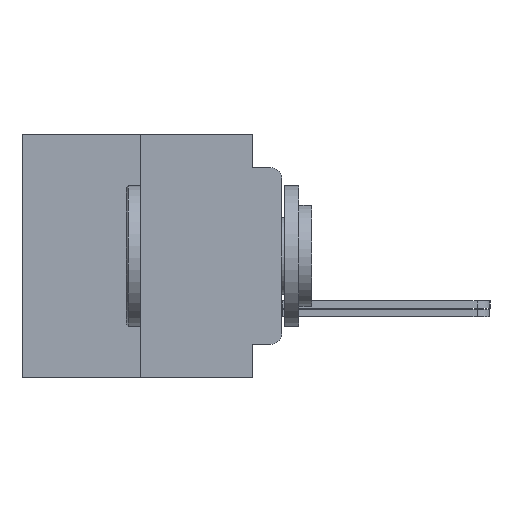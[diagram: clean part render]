
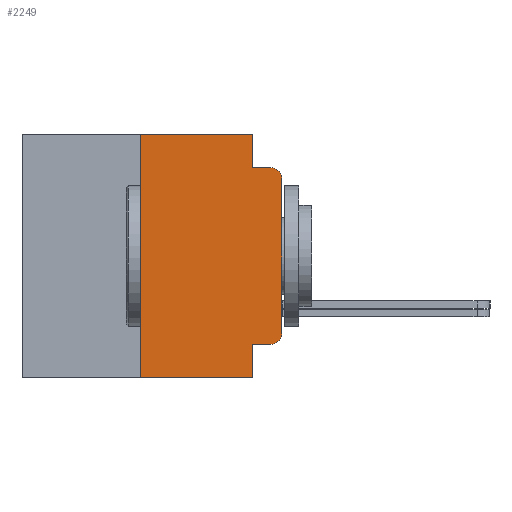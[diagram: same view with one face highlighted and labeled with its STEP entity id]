
A CAD part, left-side view. The second image highlights one B-rep face of the part: STEP entity #2249.
In plain terms, the highlighted planar face has unit normal (-1, 0, 0).
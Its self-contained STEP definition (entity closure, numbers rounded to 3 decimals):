
#635 = VECTOR ( 'NONE', #7273, 1000. ) ;
#1707 = CARTESIAN_POINT ( 'NONE',  ( -75.603, 0., -3.467 ) ) ;
#2099 = VERTEX_POINT ( 'NONE', #4735 ) ;
#2216 = VERTEX_POINT ( 'NONE', #3158 ) ;
#2249 = ADVANCED_FACE ( 'NONE', ( #16109 ), #23556, .F. ) ;
#3158 = CARTESIAN_POINT ( 'NONE',  ( -75.603, 0.508, 3.975 ) ) ;
#4472 = CARTESIAN_POINT ( 'NONE',  ( -75.603, 1.295, 0. ) ) ;
#4568 = DIRECTION ( 'NONE',  ( 0., 0., -1. ) ) ;
#4735 = CARTESIAN_POINT ( 'NONE',  ( -75.603, 1.295, 5.486 ) ) ;
#5541 = DIRECTION ( 'NONE',  ( 0., -1., 0. ) ) ;
#5819 = CARTESIAN_POINT ( 'NONE',  ( -75.603, 0., 3.467 ) ) ;
#6645 = DIRECTION ( 'NONE',  ( 1., 0., 0. ) ) ;
#6943 = CARTESIAN_POINT ( 'NONE',  ( -75.603, 1.295, -5.486 ) ) ;
#7176 = EDGE_CURVE ( 'NONE', #11286, #13524, #8114, .T. ) ;
#7273 = DIRECTION ( 'NONE',  ( 0., 0., -1. ) ) ;
#7863 = DIRECTION ( 'NONE',  ( 0., -1., 0. ) ) ;
#8114 = LINE ( 'NONE', #4472, #19538 ) ;
#8391 = CARTESIAN_POINT ( 'NONE',  ( -75.603, 6.35, -5.486 ) ) ;
#8908 = AXIS2_PLACEMENT_3D ( 'NONE', #24683, #9398, #13690 ) ;
#9398 = DIRECTION ( 'NONE',  ( -1., 0., 0. ) ) ;
#9403 = VECTOR ( 'NONE', #5541, 1000. ) ;
#9796 = VECTOR ( 'NONE', #18139, 1000. ) ;
#9869 = ORIENTED_EDGE ( 'NONE', *, *, #16320, .T. ) ;
#10389 = LINE ( 'NONE', #19634, #22148 ) ;
#10450 = LINE ( 'NONE', #12108, #10814 ) ;
#10778 = ORIENTED_EDGE ( 'NONE', *, *, #14325, .T. ) ;
#10789 = DIRECTION ( 'NONE',  ( 0., -1., 0. ) ) ;
#10814 = VECTOR ( 'NONE', #7863, 1000. ) ;
#11286 = VERTEX_POINT ( 'NONE', #19672 ) ;
#12108 = CARTESIAN_POINT ( 'NONE',  ( -75.603, 1.295, 3.975 ) ) ;
#12488 = VERTEX_POINT ( 'NONE', #27074 ) ;
#12587 = ORIENTED_EDGE ( 'NONE', *, *, #17079, .T. ) ;
#13168 = VECTOR ( 'NONE', #18884, 1000. ) ;
#13292 = DIRECTION ( 'NONE',  ( 0., 0., -1. ) ) ;
#13524 = VERTEX_POINT ( 'NONE', #6943 ) ;
#13567 = CARTESIAN_POINT ( 'NONE',  ( -75.603, 0.508, 3.467 ) ) ;
#13690 = DIRECTION ( 'NONE',  ( 0., 0., -1. ) ) ;
#13769 = CARTESIAN_POINT ( 'NONE',  ( -75.603, 1.295, 0. ) ) ;
#14325 = EDGE_CURVE ( 'NONE', #12488, #19730, #21198, .T. ) ;
#14415 = EDGE_CURVE ( 'NONE', #18753, #2216, #10450, .T. ) ;
#14769 = CARTESIAN_POINT ( 'NONE',  ( -75.603, 11.684, 5.486 ) ) ;
#15296 = LINE ( 'NONE', #22567, #9403 ) ;
#15352 = LINE ( 'NONE', #23846, #22287 ) ;
#15490 = EDGE_CURVE ( 'NONE', #19730, #21276, #24213, .T. ) ;
#15500 = DIRECTION ( 'NONE',  ( -1., 0., 0. ) ) ;
#15607 = ORIENTED_EDGE ( 'NONE', *, *, #22983, .T. ) ;
#16109 = FACE_OUTER_BOUND ( 'NONE', #23797, .T. ) ;
#16320 = EDGE_CURVE ( 'NONE', #11286, #12488, #15352, .T. ) ;
#16525 = ORIENTED_EDGE ( 'NONE', *, *, #7176, .F. ) ;
#16544 = EDGE_CURVE ( 'NONE', #26548, #2099, #24331, .T. ) ;
#16653 = ORIENTED_EDGE ( 'NONE', *, *, #18937, .F. ) ;
#17079 = EDGE_CURVE ( 'NONE', #21276, #2216, #27389, .T. ) ;
#18139 = DIRECTION ( 'NONE',  ( 0., -1., 0. ) ) ;
#18154 = AXIS2_PLACEMENT_3D ( 'NONE', #14769, #6645, #19888 ) ;
#18242 = CARTESIAN_POINT ( 'NONE',  ( -75.603, 11.684, 5.486 ) ) ;
#18753 = VERTEX_POINT ( 'NONE', #20143 ) ;
#18772 = CARTESIAN_POINT ( 'NONE',  ( -75.603, 0., 5.486 ) ) ;
#18884 = DIRECTION ( 'NONE',  ( 0., 0., 1. ) ) ;
#18937 = EDGE_CURVE ( 'NONE', #2099, #18753, #23159, .T. ) ;
#19538 = VECTOR ( 'NONE', #13292, 1000. ) ;
#19634 = CARTESIAN_POINT ( 'NONE',  ( -75.603, 6.35, -5.486 ) ) ;
#19672 = CARTESIAN_POINT ( 'NONE',  ( -75.603, 1.295, -3.975 ) ) ;
#19730 = VERTEX_POINT ( 'NONE', #1707 ) ;
#19888 = DIRECTION ( 'NONE',  ( 0., 0., -1. ) ) ;
#20110 = ORIENTED_EDGE ( 'NONE', *, *, #16544, .F. ) ;
#20143 = CARTESIAN_POINT ( 'NONE',  ( -75.603, 1.295, 3.975 ) ) ;
#21198 = CIRCLE ( 'NONE', #8908, 0.508 ) ;
#21220 = ORIENTED_EDGE ( 'NONE', *, *, #23876, .F. ) ;
#21276 = VERTEX_POINT ( 'NONE', #5819 ) ;
#21447 = ORIENTED_EDGE ( 'NONE', *, *, #14415, .F. ) ;
#22038 = DIRECTION ( 'NONE',  ( 0., 0., 1. ) ) ;
#22148 = VECTOR ( 'NONE', #22038, 1000. ) ;
#22287 = VECTOR ( 'NONE', #10789, 1000. ) ;
#22567 = CARTESIAN_POINT ( 'NONE',  ( -75.603, 11.684, -5.486 ) ) ;
#22983 = EDGE_CURVE ( 'NONE', #28380, #13524, #15296, .T. ) ;
#23159 = LINE ( 'NONE', #13769, #635 ) ;
#23556 = PLANE ( 'NONE',  #18154 ) ;
#23797 = EDGE_LOOP ( 'NONE', ( #9869, #10778, #27036, #12587, #21447, #16653, #20110, #21220, #15607, #16525 ) ) ;
#23846 = CARTESIAN_POINT ( 'NONE',  ( -75.603, 1.295, -3.975 ) ) ;
#23876 = EDGE_CURVE ( 'NONE', #28380, #26548, #10389, .T. ) ;
#24213 = LINE ( 'NONE', #18772, #13168 ) ;
#24331 = LINE ( 'NONE', #18242, #9796 ) ;
#24683 = CARTESIAN_POINT ( 'NONE',  ( -75.603, 0.508, -3.467 ) ) ;
#24698 = AXIS2_PLACEMENT_3D ( 'NONE', #13567, #15500, #4568 ) ;
#25212 = CARTESIAN_POINT ( 'NONE',  ( -75.603, 6.35, 5.486 ) ) ;
#26548 = VERTEX_POINT ( 'NONE', #25212 ) ;
#27036 = ORIENTED_EDGE ( 'NONE', *, *, #15490, .T. ) ;
#27074 = CARTESIAN_POINT ( 'NONE',  ( -75.603, 0.508, -3.975 ) ) ;
#27389 = CIRCLE ( 'NONE', #24698, 0.508 ) ;
#28380 = VERTEX_POINT ( 'NONE', #8391 ) ;
